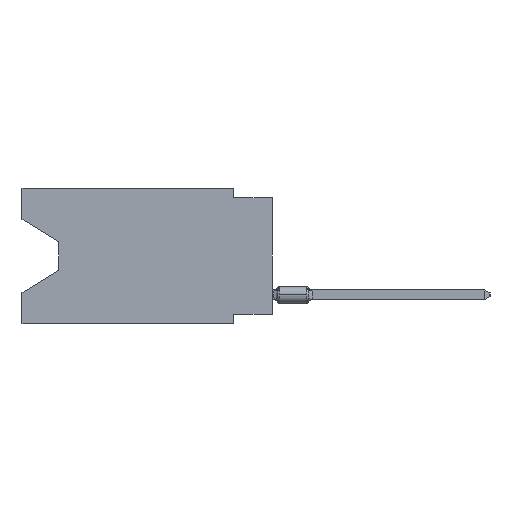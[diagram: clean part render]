
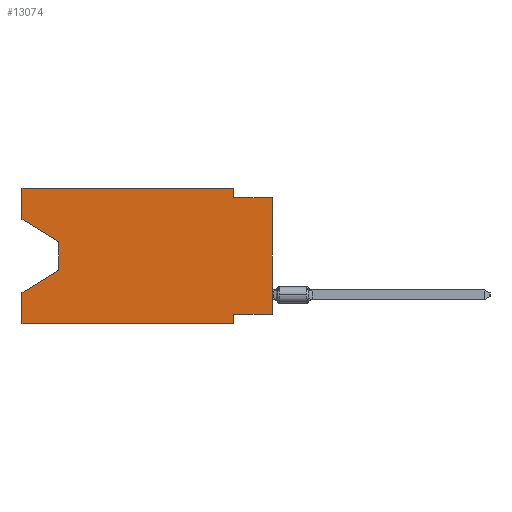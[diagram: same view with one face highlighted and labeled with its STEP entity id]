
A CAD part, left-side view. The second image highlights one B-rep face of the part: STEP entity #13074.
In plain terms, the highlighted planar face has unit normal (-1, 0, 0).
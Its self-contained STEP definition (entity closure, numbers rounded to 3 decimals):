
#32 = ORIENTED_EDGE ( 'NONE', *, *, #25766, .T. ) ;
#492 = VECTOR ( 'NONE', #9333, 1000. ) ;
#663 = LINE ( 'NONE', #18376, #5557 ) ;
#1406 = VERTEX_POINT ( 'NONE', #32391 ) ;
#1995 = ORIENTED_EDGE ( 'NONE', *, *, #21714, .T. ) ;
#2245 = VERTEX_POINT ( 'NONE', #28708 ) ;
#2675 = CARTESIAN_POINT ( 'NONE',  ( 0., 2.54, -8.255 ) ) ;
#3058 = DIRECTION ( 'NONE',  ( 0., -1., 0. ) ) ;
#3465 = CARTESIAN_POINT ( 'NONE',  ( 0., 16.383, -8.89 ) ) ;
#5250 = CARTESIAN_POINT ( 'NONE',  ( 0., 0., -8.255 ) ) ;
#5300 = CARTESIAN_POINT ( 'NONE',  ( 0., 16.383, 0. ) ) ;
#5557 = VECTOR ( 'NONE', #18777, 1000. ) ;
#6142 = VECTOR ( 'NONE', #19384, 1000. ) ;
#6522 = VECTOR ( 'NONE', #3058, 1000. ) ;
#6991 = VECTOR ( 'NONE', #19765, 1000. ) ;
#7084 = VERTEX_POINT ( 'NONE', #22156 ) ;
#7175 = VERTEX_POINT ( 'NONE', #2675 ) ;
#8363 = VECTOR ( 'NONE', #9100, 1000. ) ;
#8453 = EDGE_CURVE ( 'NONE', #34316, #29349, #35710, .T. ) ;
#8692 = EDGE_CURVE ( 'NONE', #15832, #24526, #27867, .T. ) ;
#8883 = ORIENTED_EDGE ( 'NONE', *, *, #30515, .F. ) ;
#9100 = DIRECTION ( 'NONE',  ( 0., 0., -1. ) ) ;
#9333 = DIRECTION ( 'NONE',  ( 0., -0.855, -0.519 ) ) ;
#9356 = VECTOR ( 'NONE', #13536, 1000. ) ;
#10328 = CARTESIAN_POINT ( 'NONE',  ( 0., 2.54, 0. ) ) ;
#11274 = DIRECTION ( 'NONE',  ( 0., 0., -1. ) ) ;
#11452 = ORIENTED_EDGE ( 'NONE', *, *, #26657, .F. ) ;
#12185 = DIRECTION ( 'NONE',  ( 0., -1., 0. ) ) ;
#12348 = CARTESIAN_POINT ( 'NONE',  ( 0., 16.383, -2.038 ) ) ;
#13051 = ORIENTED_EDGE ( 'NONE', *, *, #18058, .T. ) ;
#13074 = ADVANCED_FACE ( 'NONE', ( #38882 ), #35858, .F. ) ;
#13493 = EDGE_CURVE ( 'NONE', #7175, #36286, #38827, .T. ) ;
#13536 = DIRECTION ( 'NONE',  ( 0., 0., -1. ) ) ;
#14594 = CARTESIAN_POINT ( 'NONE',  ( 0., 13.97, -5.385 ) ) ;
#15570 = LINE ( 'NONE', #12348, #492 ) ;
#15832 = VERTEX_POINT ( 'NONE', #5250 ) ;
#16282 = ORIENTED_EDGE ( 'NONE', *, *, #25857, .F. ) ;
#16509 = CARTESIAN_POINT ( 'NONE',  ( 0., 13.97, -5.385 ) ) ;
#17219 = DIRECTION ( 'NONE',  ( 0., 0.855, -0.519 ) ) ;
#17558 = VERTEX_POINT ( 'NONE', #18205 ) ;
#18058 = EDGE_CURVE ( 'NONE', #17558, #36286, #25199, .T. ) ;
#18205 = CARTESIAN_POINT ( 'NONE',  ( 0., 16.383, -8.89 ) ) ;
#18376 = CARTESIAN_POINT ( 'NONE',  ( 0., 16.383, 0. ) ) ;
#18725 = ORIENTED_EDGE ( 'NONE', *, *, #8453, .T. ) ;
#18777 = DIRECTION ( 'NONE',  ( 0., -1., 0. ) ) ;
#19120 = ORIENTED_EDGE ( 'NONE', *, *, #8692, .T. ) ;
#19384 = DIRECTION ( 'NONE',  ( 0., 0., 1. ) ) ;
#19572 = CARTESIAN_POINT ( 'NONE',  ( 0., 0., -8.255 ) ) ;
#19605 = ORIENTED_EDGE ( 'NONE', *, *, #29206, .F. ) ;
#19765 = DIRECTION ( 'NONE',  ( 0., 1., 0. ) ) ;
#20133 = CARTESIAN_POINT ( 'NONE',  ( 0., 2.54, -8.89 ) ) ;
#20558 = CARTESIAN_POINT ( 'NONE',  ( 0., 16.383, -6.852 ) ) ;
#20996 = LINE ( 'NONE', #33469, #35267 ) ;
#21714 = EDGE_CURVE ( 'NONE', #2245, #34316, #36241, .T. ) ;
#21881 = CARTESIAN_POINT ( 'NONE',  ( 0., 2.54, -8.89 ) ) ;
#22062 = ORIENTED_EDGE ( 'NONE', *, *, #27050, .F. ) ;
#22074 = VERTEX_POINT ( 'NONE', #27901 ) ;
#22156 = CARTESIAN_POINT ( 'NONE',  ( 0., 2.54, 0. ) ) ;
#22599 = LINE ( 'NONE', #10328, #9356 ) ;
#22630 = DIRECTION ( 'NONE',  ( 0., 0., 1. ) ) ;
#24170 = CARTESIAN_POINT ( 'NONE',  ( 0., 13.97, -3.505 ) ) ;
#24526 = VERTEX_POINT ( 'NONE', #33164 ) ;
#24652 = LINE ( 'NONE', #39739, #37840 ) ;
#25199 = LINE ( 'NONE', #3465, #6522 ) ;
#25766 = EDGE_CURVE ( 'NONE', #22074, #2245, #15570, .T. ) ;
#25857 = EDGE_CURVE ( 'NONE', #15832, #7175, #39696, .T. ) ;
#26244 = VERTEX_POINT ( 'NONE', #27738 ) ;
#26406 = EDGE_LOOP ( 'NONE', ( #32, #1995, #18725, #22062, #13051, #39157, #16282, #19120, #11452, #19605, #8883, #39707 ) ) ;
#26657 = EDGE_CURVE ( 'NONE', #26244, #24526, #24652, .T. ) ;
#26808 = DIRECTION ( 'NONE',  ( 0., 0., -1. ) ) ;
#27050 = EDGE_CURVE ( 'NONE', #17558, #29349, #20996, .T. ) ;
#27738 = CARTESIAN_POINT ( 'NONE',  ( 0., 2.54, -0.635 ) ) ;
#27813 = AXIS2_PLACEMENT_3D ( 'NONE', #5300, #32453, #26808 ) ;
#27867 = LINE ( 'NONE', #28478, #30276 ) ;
#27901 = CARTESIAN_POINT ( 'NONE',  ( 0., 16.383, -2.038 ) ) ;
#28478 = CARTESIAN_POINT ( 'NONE',  ( 0., 0., 0. ) ) ;
#28641 = CARTESIAN_POINT ( 'NONE',  ( 0., 16.383, 0. ) ) ;
#28708 = CARTESIAN_POINT ( 'NONE',  ( 0., 13.97, -3.505 ) ) ;
#29206 = EDGE_CURVE ( 'NONE', #7084, #26244, #22599, .T. ) ;
#29349 = VERTEX_POINT ( 'NONE', #20558 ) ;
#30276 = VECTOR ( 'NONE', #22630, 1000. ) ;
#30515 = EDGE_CURVE ( 'NONE', #1406, #7084, #663, .T. ) ;
#31884 = EDGE_CURVE ( 'NONE', #22074, #1406, #34667, .T. ) ;
#32391 = CARTESIAN_POINT ( 'NONE',  ( 0., 16.383, 0. ) ) ;
#32453 = DIRECTION ( 'NONE',  ( 1., 0., 0. ) ) ;
#32968 = VECTOR ( 'NONE', #11274, 1000. ) ;
#33164 = CARTESIAN_POINT ( 'NONE',  ( 0., 0., -0.635 ) ) ;
#33469 = CARTESIAN_POINT ( 'NONE',  ( 0., 16.383, 0. ) ) ;
#33497 = VECTOR ( 'NONE', #17219, 1000. ) ;
#34316 = VERTEX_POINT ( 'NONE', #16509 ) ;
#34667 = LINE ( 'NONE', #28641, #6142 ) ;
#35267 = VECTOR ( 'NONE', #36676, 1000. ) ;
#35710 = LINE ( 'NONE', #14594, #33497 ) ;
#35858 = PLANE ( 'NONE',  #27813 ) ;
#36241 = LINE ( 'NONE', #24170, #8363 ) ;
#36286 = VERTEX_POINT ( 'NONE', #21881 ) ;
#36676 = DIRECTION ( 'NONE',  ( 0., 0., 1. ) ) ;
#37840 = VECTOR ( 'NONE', #12185, 1000. ) ;
#38827 = LINE ( 'NONE', #20133, #32968 ) ;
#38882 = FACE_OUTER_BOUND ( 'NONE', #26406, .T. ) ;
#39157 = ORIENTED_EDGE ( 'NONE', *, *, #13493, .F. ) ;
#39696 = LINE ( 'NONE', #19572, #6991 ) ;
#39707 = ORIENTED_EDGE ( 'NONE', *, *, #31884, .F. ) ;
#39739 = CARTESIAN_POINT ( 'NONE',  ( 0., 0., -0.635 ) ) ;
